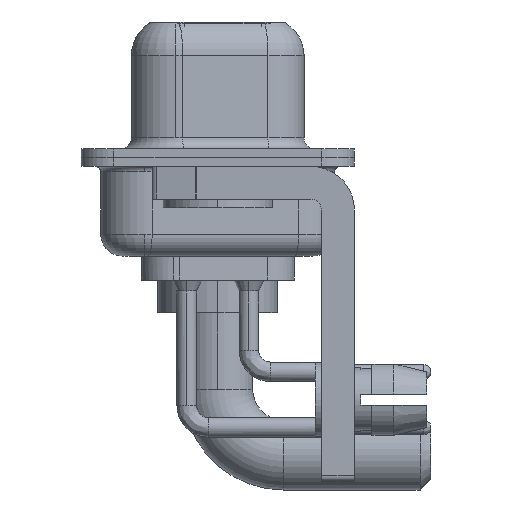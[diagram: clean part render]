
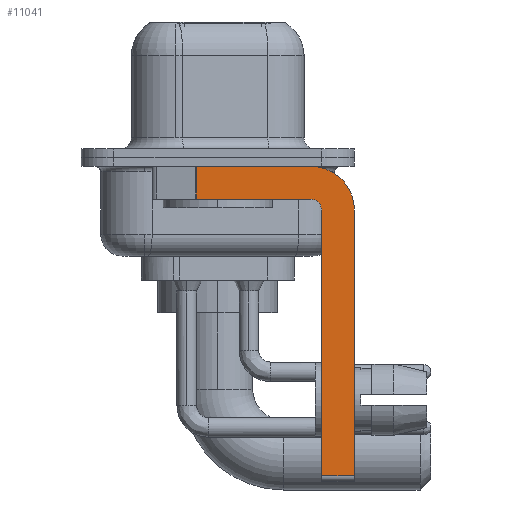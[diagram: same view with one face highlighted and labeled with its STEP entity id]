
A CAD part, left-side view. The second image highlights one B-rep face of the part: STEP entity #11041.
In plain terms, the highlighted planar face has unit normal (-1, 0, 0).
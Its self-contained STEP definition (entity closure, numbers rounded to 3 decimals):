
#413 = DIRECTION ( 'NONE',  ( 1., 0., 0. ) ) ;
#582 = ORIENTED_EDGE ( 'NONE', *, *, #6723, .F. ) ;
#693 = AXIS2_PLACEMENT_3D ( 'NONE', #17923, #14079, #8354 ) ;
#729 = VECTOR ( 'NONE', #11584, 1000. ) ;
#734 = VERTEX_POINT ( 'NONE', #23101 ) ;
#918 = FACE_OUTER_BOUND ( 'NONE', #19080, .T. ) ;
#1792 = EDGE_CURVE ( 'NONE', #19626, #734, #5211, .T. ) ;
#1817 = CARTESIAN_POINT ( 'NONE',  ( -2.9, -4.75, -14.55 ) ) ;
#1941 = CARTESIAN_POINT ( 'NONE',  ( -2.9, -4.25, -2.4 ) ) ;
#1979 = CARTESIAN_POINT ( 'NONE',  ( -2.9, -6.25, -2.4 ) ) ;
#2015 = VERTEX_POINT ( 'NONE', #1817 ) ;
#2066 = DIRECTION ( 'NONE',  ( 0., 0., -1. ) ) ;
#2127 = VECTOR ( 'NONE', #11168, 1000. ) ;
#2742 = VECTOR ( 'NONE', #11105, 1000. ) ;
#3532 = EDGE_CURVE ( 'NONE', #19692, #14214, #14668, .T. ) ;
#3913 = AXIS2_PLACEMENT_3D ( 'NONE', #21950, #9993, #6199 ) ;
#4323 = CARTESIAN_POINT ( 'NONE',  ( -2.9, -4.25, -14.55 ) ) ;
#4553 = VERTEX_POINT ( 'NONE', #20976 ) ;
#5211 = LINE ( 'NONE', #24623, #2127 ) ;
#5576 = LINE ( 'NONE', #9492, #11841 ) ;
#5652 = LINE ( 'NONE', #20779, #2742 ) ;
#6199 = DIRECTION ( 'NONE',  ( 0., 0., 1. ) ) ;
#6723 = EDGE_CURVE ( 'NONE', #14214, #23585, #22649, .T. ) ;
#8354 = DIRECTION ( 'NONE',  ( 0., 0., -1. ) ) ;
#8357 = LINE ( 'NONE', #4323, #10434 ) ;
#9241 = CARTESIAN_POINT ( 'NONE',  ( -2.9, -4.25, -1.9 ) ) ;
#9492 = CARTESIAN_POINT ( 'NONE',  ( -2.9, 0.978, -1.9 ) ) ;
#9993 = DIRECTION ( 'NONE',  ( -1., 0., 0. ) ) ;
#10145 = PLANE ( 'NONE',  #693 ) ;
#10219 = AXIS2_PLACEMENT_3D ( 'NONE', #1941, #413, #2066 ) ;
#10434 = VECTOR ( 'NONE', #10517, 1000. ) ;
#10517 = DIRECTION ( 'NONE',  ( 0., -1., 0. ) ) ;
#11041 = ADVANCED_FACE ( 'NONE', ( #918 ), #10145, .F. ) ;
#11105 = DIRECTION ( 'NONE',  ( 0., 0., 1. ) ) ;
#11168 = DIRECTION ( 'NONE',  ( 0., 1., 0. ) ) ;
#11185 = CIRCLE ( 'NONE', #3913, 0.5 ) ;
#11584 = DIRECTION ( 'NONE',  ( 0., 0., -1. ) ) ;
#11841 = VECTOR ( 'NONE', #15338, 1000. ) ;
#12341 = EDGE_CURVE ( 'NONE', #2015, #23585, #8357, .T. ) ;
#12919 = ORIENTED_EDGE ( 'NONE', *, *, #14248, .F. ) ;
#13018 = ORIENTED_EDGE ( 'NONE', *, *, #3532, .F. ) ;
#14079 = DIRECTION ( 'NONE',  ( 1., 0., 0. ) ) ;
#14214 = VERTEX_POINT ( 'NONE', #21689 ) ;
#14248 = EDGE_CURVE ( 'NONE', #4553, #19692, #14791, .T. ) ;
#14371 = ORIENTED_EDGE ( 'NONE', *, *, #21971, .F. ) ;
#14668 = CIRCLE ( 'NONE', #10219, 2. ) ;
#14671 = DIRECTION ( 'NONE',  ( 0., -1., 0. ) ) ;
#14791 = LINE ( 'NONE', #18483, #20264 ) ;
#15106 = ORIENTED_EDGE ( 'NONE', *, *, #18204, .T. ) ;
#15338 = DIRECTION ( 'NONE',  ( 0., 0., -1. ) ) ;
#15696 = CARTESIAN_POINT ( 'NONE',  ( -2.9, -6.25, -14.55 ) ) ;
#16008 = ORIENTED_EDGE ( 'NONE', *, *, #12341, .T. ) ;
#16793 = ORIENTED_EDGE ( 'NONE', *, *, #22772, .F. ) ;
#17329 = ORIENTED_EDGE ( 'NONE', *, *, #1792, .F. ) ;
#17923 = CARTESIAN_POINT ( 'NONE',  ( -2.9, -4.25, -2.4 ) ) ;
#18204 = EDGE_CURVE ( 'NONE', #4553, #734, #5576, .T. ) ;
#18483 = CARTESIAN_POINT ( 'NONE',  ( -2.9, 3., -0.4 ) ) ;
#18607 = VERTEX_POINT ( 'NONE', #23937 ) ;
#19080 = EDGE_LOOP ( 'NONE', ( #12919, #15106, #17329, #14371, #16793, #16008, #582, #13018 ) ) ;
#19626 = VERTEX_POINT ( 'NONE', #9241 ) ;
#19692 = VERTEX_POINT ( 'NONE', #24863 ) ;
#20264 = VECTOR ( 'NONE', #14671, 1000. ) ;
#20779 = CARTESIAN_POINT ( 'NONE',  ( -2.9, -4.75, -14.8 ) ) ;
#20976 = CARTESIAN_POINT ( 'NONE',  ( -2.9, 0.978, -0.4 ) ) ;
#21689 = CARTESIAN_POINT ( 'NONE',  ( -2.9, -6.25, -2.4 ) ) ;
#21950 = CARTESIAN_POINT ( 'NONE',  ( -2.9, -4.25, -2.4 ) ) ;
#21971 = EDGE_CURVE ( 'NONE', #18607, #19626, #11185, .T. ) ;
#22649 = LINE ( 'NONE', #1979, #729 ) ;
#22772 = EDGE_CURVE ( 'NONE', #2015, #18607, #5652, .T. ) ;
#23101 = CARTESIAN_POINT ( 'NONE',  ( -2.9, 0.978, -1.9 ) ) ;
#23585 = VERTEX_POINT ( 'NONE', #15696 ) ;
#23937 = CARTESIAN_POINT ( 'NONE',  ( -2.9, -4.75, -2.4 ) ) ;
#24623 = CARTESIAN_POINT ( 'NONE',  ( -2.9, -4.25, -1.9 ) ) ;
#24863 = CARTESIAN_POINT ( 'NONE',  ( -2.9, -4.25, -0.4 ) ) ;
